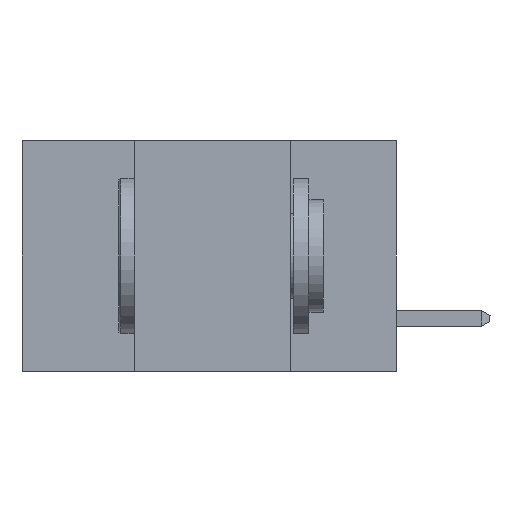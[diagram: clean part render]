
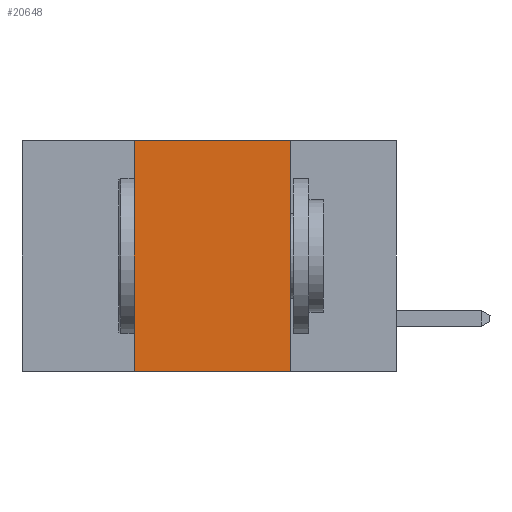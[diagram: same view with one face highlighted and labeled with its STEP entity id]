
A CAD part, left-side view. The second image highlights one B-rep face of the part: STEP entity #20648.
In plain terms, the highlighted planar face has unit normal (-1, 0, 0).
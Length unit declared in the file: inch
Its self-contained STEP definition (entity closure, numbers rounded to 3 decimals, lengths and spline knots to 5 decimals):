
#345 = VECTOR ( 'NONE', #10306, 39.37008 ) ;
#667 = PLANE ( 'NONE',  #4069 ) ;
#1699 = CARTESIAN_POINT ( 'NONE',  ( 0., 0.42, -0.37 ) ) ;
#2288 = CARTESIAN_POINT ( 'NONE',  ( 0., 0.42, 0. ) ) ;
#2332 = DIRECTION ( 'NONE',  ( 0., 0., -1. ) ) ;
#2589 = CARTESIAN_POINT ( 'NONE',  ( 0., 0.17, -0.37 ) ) ;
#2848 = EDGE_LOOP ( 'NONE', ( #10433, #18926, #10922, #15699 ) ) ;
#2945 = CARTESIAN_POINT ( 'NONE',  ( 0., 0.6, 0. ) ) ;
#3684 = CARTESIAN_POINT ( 'NONE',  ( 0., 0.42, -0.37 ) ) ;
#3792 = LINE ( 'NONE', #1699, #19774 ) ;
#3963 = LINE ( 'NONE', #2945, #20404 ) ;
#4069 = AXIS2_PLACEMENT_3D ( 'NONE', #7088, #11981, #2332 ) ;
#4175 = CARTESIAN_POINT ( 'NONE',  ( 0., 0.6, -0.37 ) ) ;
#4776 = LINE ( 'NONE', #4175, #17618 ) ;
#4795 = VERTEX_POINT ( 'NONE', #2288 ) ;
#5679 = DIRECTION ( 'NONE',  ( 0., -1., 0. ) ) ;
#6057 = DIRECTION ( 'NONE',  ( 0., -1., 0. ) ) ;
#7088 = CARTESIAN_POINT ( 'NONE',  ( 0., 0.6, 0. ) ) ;
#7166 = VERTEX_POINT ( 'NONE', #2589 ) ;
#8477 = LINE ( 'NONE', #19802, #345 ) ;
#9902 = EDGE_CURVE ( 'NONE', #15204, #7166, #4776, .T. ) ;
#10306 = DIRECTION ( 'NONE',  ( 0., 0., -1. ) ) ;
#10433 = ORIENTED_EDGE ( 'NONE', *, *, #15277, .F. ) ;
#10922 = ORIENTED_EDGE ( 'NONE', *, *, #12030, .F. ) ;
#11384 = VERTEX_POINT ( 'NONE', #15994 ) ;
#11981 = DIRECTION ( 'NONE',  ( 1., 0., 0. ) ) ;
#12030 = EDGE_CURVE ( 'NONE', #15204, #4795, #3792, .T. ) ;
#14214 = EDGE_CURVE ( 'NONE', #4795, #11384, #3963, .T. ) ;
#14596 = DIRECTION ( 'NONE',  ( 0., 0., 1. ) ) ;
#15204 = VERTEX_POINT ( 'NONE', #3684 ) ;
#15277 = EDGE_CURVE ( 'NONE', #11384, #7166, #8477, .T. ) ;
#15699 = ORIENTED_EDGE ( 'NONE', *, *, #9902, .T. ) ;
#15994 = CARTESIAN_POINT ( 'NONE',  ( 0., 0.17, 0. ) ) ;
#17618 = VECTOR ( 'NONE', #5679, 39.37008 ) ;
#17897 = FACE_OUTER_BOUND ( 'NONE', #2848, .T. ) ;
#18926 = ORIENTED_EDGE ( 'NONE', *, *, #14214, .F. ) ;
#19774 = VECTOR ( 'NONE', #14596, 39.37008 ) ;
#19802 = CARTESIAN_POINT ( 'NONE',  ( 0., 0.17, -0.37 ) ) ;
#20404 = VECTOR ( 'NONE', #6057, 39.37008 ) ;
#20648 = ADVANCED_FACE ( 'NONE', ( #17897 ), #667, .F. ) ;
